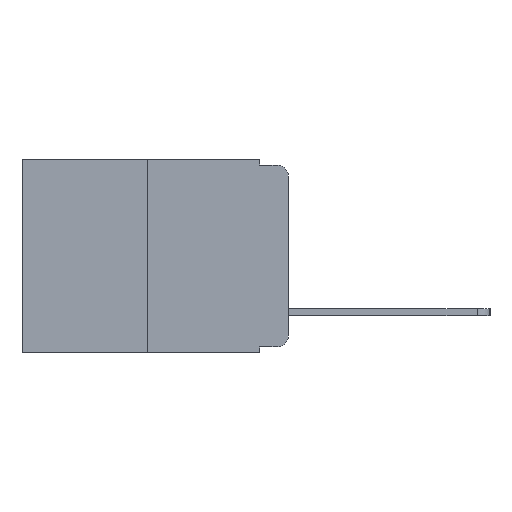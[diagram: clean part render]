
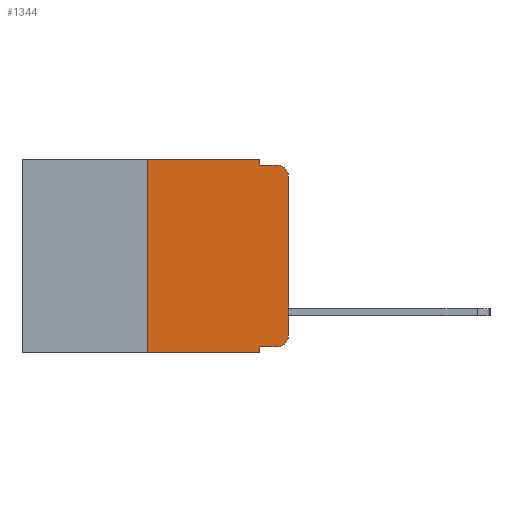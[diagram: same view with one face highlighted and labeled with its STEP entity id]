
A CAD part, left-side view. The second image highlights one B-rep face of the part: STEP entity #1344.
In plain terms, the highlighted planar face has unit normal (-1, 0, 0).
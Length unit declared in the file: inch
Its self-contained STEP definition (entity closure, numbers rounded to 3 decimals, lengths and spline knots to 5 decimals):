
#70 = CARTESIAN_POINT ( 'NONE',  ( 0., 0.051, -0.343 ) ) ;
#93 = ORIENTED_EDGE ( 'NONE', *, *, #4174, .F. ) ;
#156 = CARTESIAN_POINT ( 'NONE',  ( 0., 0.473, -0.343 ) ) ;
#371 = VECTOR ( 'NONE', #12366, 39.37008 ) ;
#376 = VERTEX_POINT ( 'NONE', #8388 ) ;
#859 = EDGE_CURVE ( 'NONE', #11912, #3435, #4678, .T. ) ;
#1226 = VERTEX_POINT ( 'NONE', #9175 ) ;
#1297 = EDGE_CURVE ( 'NONE', #1226, #11912, #12254, .T. ) ;
#1316 = DIRECTION ( 'NONE',  ( 0., -1., 0. ) ) ;
#1344 = ADVANCED_FACE ( 'NONE', ( #9135 ), #11978, .F. ) ;
#1363 = ORIENTED_EDGE ( 'NONE', *, *, #859, .T. ) ;
#1491 = LINE ( 'NONE', #2228, #11104 ) ;
#1531 = CARTESIAN_POINT ( 'NONE',  ( 0., 0., 0. ) ) ;
#1623 = VECTOR ( 'NONE', #10124, 39.37008 ) ;
#1724 = VECTOR ( 'NONE', #11106, 39.37008 ) ;
#1927 = CARTESIAN_POINT ( 'NONE',  ( 0., 0.02, -0.01 ) ) ;
#2044 = LINE ( 'NONE', #6642, #1724 ) ;
#2228 = CARTESIAN_POINT ( 'NONE',  ( 0., 0.473, 0. ) ) ;
#2393 = LINE ( 'NONE', #11702, #7143 ) ;
#2576 = EDGE_CURVE ( 'NONE', #1226, #7581, #9226, .T. ) ;
#2720 = EDGE_CURVE ( 'NONE', #376, #7044, #3335, .T. ) ;
#2772 = CIRCLE ( 'NONE', #7545, 0.02 ) ;
#2827 = CARTESIAN_POINT ( 'NONE',  ( 0., 0., -0.313 ) ) ;
#2921 = EDGE_CURVE ( 'NONE', #9490, #4980, #2772, .T. ) ;
#3059 = ORIENTED_EDGE ( 'NONE', *, *, #2720, .F. ) ;
#3335 = LINE ( 'NONE', #7024, #371 ) ;
#3435 = VERTEX_POINT ( 'NONE', #2827 ) ;
#3576 = DIRECTION ( 'NONE',  ( 0., -1., 0. ) ) ;
#3673 = DIRECTION ( 'NONE',  ( -1., 0., 0. ) ) ;
#3721 = DIRECTION ( 'NONE',  ( 1., 0., 0. ) ) ;
#3845 = EDGE_CURVE ( 'NONE', #6452, #7581, #7866, .T. ) ;
#4174 = EDGE_CURVE ( 'NONE', #7044, #4980, #2393, .T. ) ;
#4300 = CARTESIAN_POINT ( 'NONE',  ( 0., 0., -0.03 ) ) ;
#4678 = CIRCLE ( 'NONE', #9600, 0.02 ) ;
#4980 = VERTEX_POINT ( 'NONE', #1927 ) ;
#5476 = ORIENTED_EDGE ( 'NONE', *, *, #6382, .T. ) ;
#5752 = CARTESIAN_POINT ( 'NONE',  ( 0., 0.25, -0.343 ) ) ;
#6035 = ORIENTED_EDGE ( 'NONE', *, *, #6172, .F. ) ;
#6172 = EDGE_CURVE ( 'NONE', #9783, #376, #1491, .T. ) ;
#6375 = DIRECTION ( 'NONE',  ( -1., 0., 0. ) ) ;
#6382 = EDGE_CURVE ( 'NONE', #3435, #9490, #6468, .T. ) ;
#6392 = DIRECTION ( 'NONE',  ( 0., 0., -1. ) ) ;
#6452 = VERTEX_POINT ( 'NONE', #5752 ) ;
#6468 = LINE ( 'NONE', #1531, #10693 ) ;
#6544 = CARTESIAN_POINT ( 'NONE',  ( 0., 0.051, -0.01 ) ) ;
#6602 = DIRECTION ( 'NONE',  ( 0., 0., 1. ) ) ;
#6642 = CARTESIAN_POINT ( 'NONE',  ( 0., 0.25, 0. ) ) ;
#7024 = CARTESIAN_POINT ( 'NONE',  ( 0., 0.051, 0. ) ) ;
#7044 = VERTEX_POINT ( 'NONE', #6544 ) ;
#7143 = VECTOR ( 'NONE', #8362, 39.37008 ) ;
#7464 = CARTESIAN_POINT ( 'NONE',  ( 0., 0.051, 0. ) ) ;
#7545 = AXIS2_PLACEMENT_3D ( 'NONE', #9356, #3673, #10232 ) ;
#7566 = AXIS2_PLACEMENT_3D ( 'NONE', #10233, #3721, #10265 ) ;
#7581 = VERTEX_POINT ( 'NONE', #70 ) ;
#7850 = ORIENTED_EDGE ( 'NONE', *, *, #2576, .F. ) ;
#7866 = LINE ( 'NONE', #156, #12285 ) ;
#7981 = ORIENTED_EDGE ( 'NONE', *, *, #2921, .T. ) ;
#8189 = CARTESIAN_POINT ( 'NONE',  ( 0., 0.02, -0.333 ) ) ;
#8359 = CARTESIAN_POINT ( 'NONE',  ( 0., 0.051, -0.333 ) ) ;
#8362 = DIRECTION ( 'NONE',  ( 0., -1., 0. ) ) ;
#8388 = CARTESIAN_POINT ( 'NONE',  ( 0., 0.051, 0. ) ) ;
#8445 = EDGE_LOOP ( 'NONE', ( #5476, #7981, #93, #3059, #6035, #11128, #9146, #7850, #12531, #1363 ) ) ;
#9135 = FACE_OUTER_BOUND ( 'NONE', #8445, .T. ) ;
#9146 = ORIENTED_EDGE ( 'NONE', *, *, #3845, .T. ) ;
#9175 = CARTESIAN_POINT ( 'NONE',  ( 0., 0.051, -0.333 ) ) ;
#9226 = LINE ( 'NONE', #7464, #1623 ) ;
#9356 = CARTESIAN_POINT ( 'NONE',  ( 0., 0.02, -0.03 ) ) ;
#9490 = VERTEX_POINT ( 'NONE', #4300 ) ;
#9600 = AXIS2_PLACEMENT_3D ( 'NONE', #12360, #6375, #6392 ) ;
#9783 = VERTEX_POINT ( 'NONE', #10110 ) ;
#9951 = VECTOR ( 'NONE', #3576, 39.37008 ) ;
#10018 = DIRECTION ( 'NONE',  ( 0., -1., 0. ) ) ;
#10110 = CARTESIAN_POINT ( 'NONE',  ( 0., 0.25, 0. ) ) ;
#10124 = DIRECTION ( 'NONE',  ( 0., 0., -1. ) ) ;
#10232 = DIRECTION ( 'NONE',  ( 0., 0., -1. ) ) ;
#10233 = CARTESIAN_POINT ( 'NONE',  ( 0., 0.473, 0. ) ) ;
#10265 = DIRECTION ( 'NONE',  ( 0., 0., -1. ) ) ;
#10693 = VECTOR ( 'NONE', #6602, 39.37008 ) ;
#11104 = VECTOR ( 'NONE', #10018, 39.37008 ) ;
#11106 = DIRECTION ( 'NONE',  ( 0., 0., 1. ) ) ;
#11128 = ORIENTED_EDGE ( 'NONE', *, *, #12155, .F. ) ;
#11702 = CARTESIAN_POINT ( 'NONE',  ( 0., 0.051, -0.01 ) ) ;
#11912 = VERTEX_POINT ( 'NONE', #8189 ) ;
#11978 = PLANE ( 'NONE',  #7566 ) ;
#12155 = EDGE_CURVE ( 'NONE', #6452, #9783, #2044, .T. ) ;
#12254 = LINE ( 'NONE', #8359, #9951 ) ;
#12285 = VECTOR ( 'NONE', #1316, 39.37008 ) ;
#12360 = CARTESIAN_POINT ( 'NONE',  ( 0., 0.02, -0.313 ) ) ;
#12366 = DIRECTION ( 'NONE',  ( 0., 0., -1. ) ) ;
#12531 = ORIENTED_EDGE ( 'NONE', *, *, #1297, .T. ) ;
